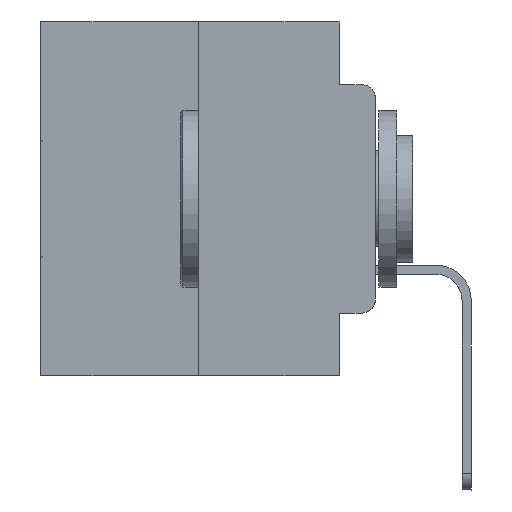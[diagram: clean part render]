
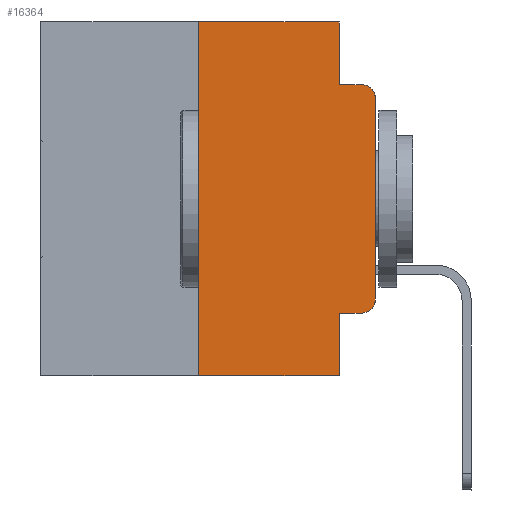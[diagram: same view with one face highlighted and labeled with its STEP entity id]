
A CAD part, left-side view. The second image highlights one B-rep face of the part: STEP entity #16364.
In plain terms, the highlighted planar face has unit normal (-1, 0, 0).
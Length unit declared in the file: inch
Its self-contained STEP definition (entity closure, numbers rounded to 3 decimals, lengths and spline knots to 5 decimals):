
#653 = EDGE_CURVE ( 'NONE', #24153, #28513, #12457, .T. ) ;
#669 = VERTEX_POINT ( 'NONE', #10586 ) ;
#828 = CARTESIAN_POINT ( 'NONE',  ( 0., 0.02, -0.4115 ) ) ;
#1299 = EDGE_CURVE ( 'NONE', #2529, #8949, #30178, .T. ) ;
#1715 = DIRECTION ( 'NONE',  ( -1., 0., 0. ) ) ;
#1804 = VECTOR ( 'NONE', #24759, 39.37008 ) ;
#2226 = VECTOR ( 'NONE', #20598, 39.37008 ) ;
#2501 = CARTESIAN_POINT ( 'NONE',  ( 0., 0.051, -0.5 ) ) ;
#2529 = VERTEX_POINT ( 'NONE', #30000 ) ;
#2548 = LINE ( 'NONE', #12783, #1804 ) ;
#2818 = CARTESIAN_POINT ( 'NONE',  ( 0., 0.473, -0.5 ) ) ;
#3307 = CARTESIAN_POINT ( 'NONE',  ( 0., 0.051, -0.0885 ) ) ;
#3456 = VECTOR ( 'NONE', #25531, 39.37008 ) ;
#3778 = ORIENTED_EDGE ( 'NONE', *, *, #22384, .F. ) ;
#4146 = LINE ( 'NONE', #21664, #12968 ) ;
#4184 = VERTEX_POINT ( 'NONE', #7965 ) ;
#4873 = ORIENTED_EDGE ( 'NONE', *, *, #11983, .T. ) ;
#5121 = VECTOR ( 'NONE', #10395, 39.37008 ) ;
#5251 = VERTEX_POINT ( 'NONE', #2501 ) ;
#5488 = FACE_OUTER_BOUND ( 'NONE', #20398, .T. ) ;
#7502 = EDGE_CURVE ( 'NONE', #14878, #24153, #8203, .T. ) ;
#7965 = CARTESIAN_POINT ( 'NONE',  ( 0., 0.051, -0.4115 ) ) ;
#8062 = VERTEX_POINT ( 'NONE', #25586 ) ;
#8203 = CIRCLE ( 'NONE', #17322, 0.02 ) ;
#8949 = VERTEX_POINT ( 'NONE', #27512 ) ;
#10395 = DIRECTION ( 'NONE',  ( 0., 0., 1. ) ) ;
#10586 = CARTESIAN_POINT ( 'NONE',  ( 0., 0.02, -0.0885 ) ) ;
#10638 = CARTESIAN_POINT ( 'NONE',  ( 0., 0., -0.3915 ) ) ;
#11056 = DIRECTION ( 'NONE',  ( 0., -1., 0. ) ) ;
#11152 = EDGE_CURVE ( 'NONE', #2529, #5251, #27265, .T. ) ;
#11983 = EDGE_CURVE ( 'NONE', #28513, #669, #17931, .T. ) ;
#12240 = DIRECTION ( 'NONE',  ( 0., -1., 0. ) ) ;
#12457 = LINE ( 'NONE', #24779, #5121 ) ;
#12763 = DIRECTION ( 'NONE',  ( 0., 0., 1. ) ) ;
#12783 = CARTESIAN_POINT ( 'NONE',  ( 0., 0.051, 0. ) ) ;
#12968 = VECTOR ( 'NONE', #26303, 39.37008 ) ;
#13551 = VECTOR ( 'NONE', #12763, 39.37008 ) ;
#14751 = LINE ( 'NONE', #22878, #2226 ) ;
#14806 = EDGE_CURVE ( 'NONE', #4184, #14878, #4146, .T. ) ;
#14878 = VERTEX_POINT ( 'NONE', #828 ) ;
#14896 = ORIENTED_EDGE ( 'NONE', *, *, #19309, .F. ) ;
#15831 = CARTESIAN_POINT ( 'NONE',  ( 0., 0.02, -0.1085 ) ) ;
#15979 = ORIENTED_EDGE ( 'NONE', *, *, #7502, .T. ) ;
#16069 = DIRECTION ( 'NONE',  ( -1., 0., 0. ) ) ;
#16185 = AXIS2_PLACEMENT_3D ( 'NONE', #18173, #20317, #20428 ) ;
#16265 = EDGE_CURVE ( 'NONE', #16834, #8062, #2548, .T. ) ;
#16364 = ADVANCED_FACE ( 'NONE', ( #5488 ), #18074, .F. ) ;
#16720 = LINE ( 'NONE', #23175, #3456 ) ;
#16834 = VERTEX_POINT ( 'NONE', #28765 ) ;
#17322 = AXIS2_PLACEMENT_3D ( 'NONE', #20713, #16069, #18448 ) ;
#17816 = ORIENTED_EDGE ( 'NONE', *, *, #11152, .T. ) ;
#17931 = CIRCLE ( 'NONE', #19001, 0.02 ) ;
#18074 = PLANE ( 'NONE',  #16185 ) ;
#18173 = CARTESIAN_POINT ( 'NONE',  ( 0., 0.473, 0. ) ) ;
#18198 = ORIENTED_EDGE ( 'NONE', *, *, #1299, .F. ) ;
#18448 = DIRECTION ( 'NONE',  ( 0., 0., -1. ) ) ;
#18664 = ORIENTED_EDGE ( 'NONE', *, *, #14806, .T. ) ;
#19001 = AXIS2_PLACEMENT_3D ( 'NONE', #15831, #1715, #30187 ) ;
#19309 = EDGE_CURVE ( 'NONE', #4184, #5251, #16720, .T. ) ;
#20317 = DIRECTION ( 'NONE',  ( 1., 0., 0. ) ) ;
#20398 = EDGE_LOOP ( 'NONE', ( #22783, #4873, #3778, #23947, #21260, #18198, #17816, #14896, #18664, #15979 ) ) ;
#20428 = DIRECTION ( 'NONE',  ( 0., 0., -1. ) ) ;
#20598 = DIRECTION ( 'NONE',  ( 0., -1., 0. ) ) ;
#20713 = CARTESIAN_POINT ( 'NONE',  ( 0., 0.02, -0.3915 ) ) ;
#21260 = ORIENTED_EDGE ( 'NONE', *, *, #26551, .F. ) ;
#21664 = CARTESIAN_POINT ( 'NONE',  ( 0., 0.051, -0.4115 ) ) ;
#21727 = VECTOR ( 'NONE', #12240, 39.37008 ) ;
#22384 = EDGE_CURVE ( 'NONE', #8062, #669, #27537, .T. ) ;
#22491 = CARTESIAN_POINT ( 'NONE',  ( 0., 0.25, 0. ) ) ;
#22783 = ORIENTED_EDGE ( 'NONE', *, *, #653, .T. ) ;
#22878 = CARTESIAN_POINT ( 'NONE',  ( 0., 0.473, 0. ) ) ;
#23175 = CARTESIAN_POINT ( 'NONE',  ( 0., 0.051, 0. ) ) ;
#23339 = CARTESIAN_POINT ( 'NONE',  ( 0., 0., -0.1085 ) ) ;
#23947 = ORIENTED_EDGE ( 'NONE', *, *, #16265, .F. ) ;
#24153 = VERTEX_POINT ( 'NONE', #10638 ) ;
#24759 = DIRECTION ( 'NONE',  ( 0., 0., -1. ) ) ;
#24779 = CARTESIAN_POINT ( 'NONE',  ( 0., 0., 0. ) ) ;
#25531 = DIRECTION ( 'NONE',  ( 0., 0., -1. ) ) ;
#25586 = CARTESIAN_POINT ( 'NONE',  ( 0., 0.051, -0.0885 ) ) ;
#26303 = DIRECTION ( 'NONE',  ( 0., -1., 0. ) ) ;
#26551 = EDGE_CURVE ( 'NONE', #8949, #16834, #14751, .T. ) ;
#27265 = LINE ( 'NONE', #2818, #21727 ) ;
#27512 = CARTESIAN_POINT ( 'NONE',  ( 0., 0.25, 0. ) ) ;
#27537 = LINE ( 'NONE', #3307, #28669 ) ;
#28513 = VERTEX_POINT ( 'NONE', #23339 ) ;
#28669 = VECTOR ( 'NONE', #11056, 39.37008 ) ;
#28765 = CARTESIAN_POINT ( 'NONE',  ( 0., 0.051, 0. ) ) ;
#30000 = CARTESIAN_POINT ( 'NONE',  ( 0., 0.25, -0.5 ) ) ;
#30178 = LINE ( 'NONE', #22491, #13551 ) ;
#30187 = DIRECTION ( 'NONE',  ( 0., 0., -1. ) ) ;
